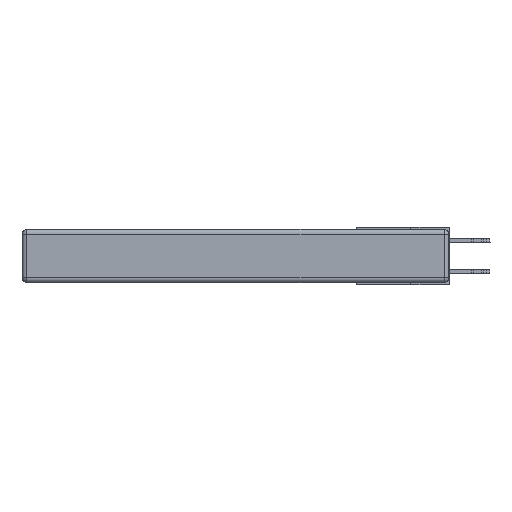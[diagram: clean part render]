
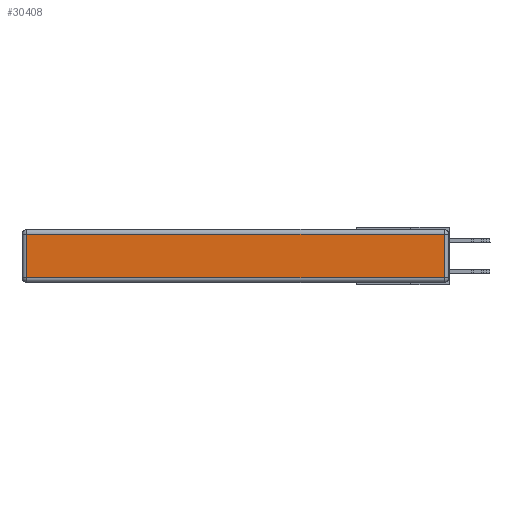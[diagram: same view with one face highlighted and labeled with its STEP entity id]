
A CAD part, left-side view. The second image highlights one B-rep face of the part: STEP entity #30408.
In plain terms, the highlighted planar face has unit normal (-1, 0, 0).
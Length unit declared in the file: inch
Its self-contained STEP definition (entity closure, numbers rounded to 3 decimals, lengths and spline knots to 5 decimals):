
#336 = FACE_OUTER_BOUND ( 'NONE', #10833, .T. ) ;
#521 = DIRECTION ( 'NONE',  ( 0., 0., 1. ) ) ;
#856 = DIRECTION ( 'NONE',  ( -1., 0., 0. ) ) ;
#1493 = CARTESIAN_POINT ( 'NONE',  ( 0., 2.72, -0.343 ) ) ;
#1645 = ORIENTED_EDGE ( 'NONE', *, *, #18864, .T. ) ;
#2639 = VERTEX_POINT ( 'NONE', #28282 ) ;
#3275 = CARTESIAN_POINT ( 'NONE',  ( 0., 0.03, -0.313 ) ) ;
#4856 = DIRECTION ( 'NONE',  ( 0., -1., 0. ) ) ;
#5659 = CARTESIAN_POINT ( 'NONE',  ( 0., 0.03, -0.343 ) ) ;
#8198 = CARTESIAN_POINT ( 'NONE',  ( 0., 2.72, -0.03 ) ) ;
#8593 = VECTOR ( 'NONE', #20021, 39.37008 ) ;
#9134 = VECTOR ( 'NONE', #13337, 39.37008 ) ;
#10833 = EDGE_LOOP ( 'NONE', ( #20578, #24351, #1645, #30068 ) ) ;
#11549 = LINE ( 'NONE', #1493, #28014 ) ;
#11577 = EDGE_CURVE ( 'NONE', #20807, #2639, #14464, .T. ) ;
#11876 = EDGE_CURVE ( 'NONE', #33292, #17844, #11549, .T. ) ;
#13337 = DIRECTION ( 'NONE',  ( 0., 0., 1. ) ) ;
#14464 = LINE ( 'NONE', #5659, #9134 ) ;
#15682 = PLANE ( 'NONE',  #22511 ) ;
#17344 = CARTESIAN_POINT ( 'NONE',  ( 0., 0., -0.313 ) ) ;
#17844 = VERTEX_POINT ( 'NONE', #23597 ) ;
#17991 = VECTOR ( 'NONE', #4856, 39.37008 ) ;
#18864 = EDGE_CURVE ( 'NONE', #2639, #33292, #24175, .T. ) ;
#18892 = CARTESIAN_POINT ( 'NONE',  ( 0., 0., -0.343 ) ) ;
#20021 = DIRECTION ( 'NONE',  ( 0., 1., 0. ) ) ;
#20578 = ORIENTED_EDGE ( 'NONE', *, *, #27579, .T. ) ;
#20807 = VERTEX_POINT ( 'NONE', #3275 ) ;
#22511 = AXIS2_PLACEMENT_3D ( 'NONE', #18892, #856, #521 ) ;
#23101 = CARTESIAN_POINT ( 'NONE',  ( 0., 2.75, -0.03 ) ) ;
#23597 = CARTESIAN_POINT ( 'NONE',  ( 0., 2.72, -0.313 ) ) ;
#24175 = LINE ( 'NONE', #23101, #8593 ) ;
#24351 = ORIENTED_EDGE ( 'NONE', *, *, #11577, .T. ) ;
#27579 = EDGE_CURVE ( 'NONE', #17844, #20807, #31917, .T. ) ;
#28014 = VECTOR ( 'NONE', #29279, 39.37008 ) ;
#28282 = CARTESIAN_POINT ( 'NONE',  ( 0., 0.03, -0.03 ) ) ;
#29279 = DIRECTION ( 'NONE',  ( 0., 0., -1. ) ) ;
#30068 = ORIENTED_EDGE ( 'NONE', *, *, #11876, .T. ) ;
#30408 = ADVANCED_FACE ( 'NONE', ( #336 ), #15682, .T. ) ;
#31917 = LINE ( 'NONE', #17344, #17991 ) ;
#33292 = VERTEX_POINT ( 'NONE', #8198 ) ;
